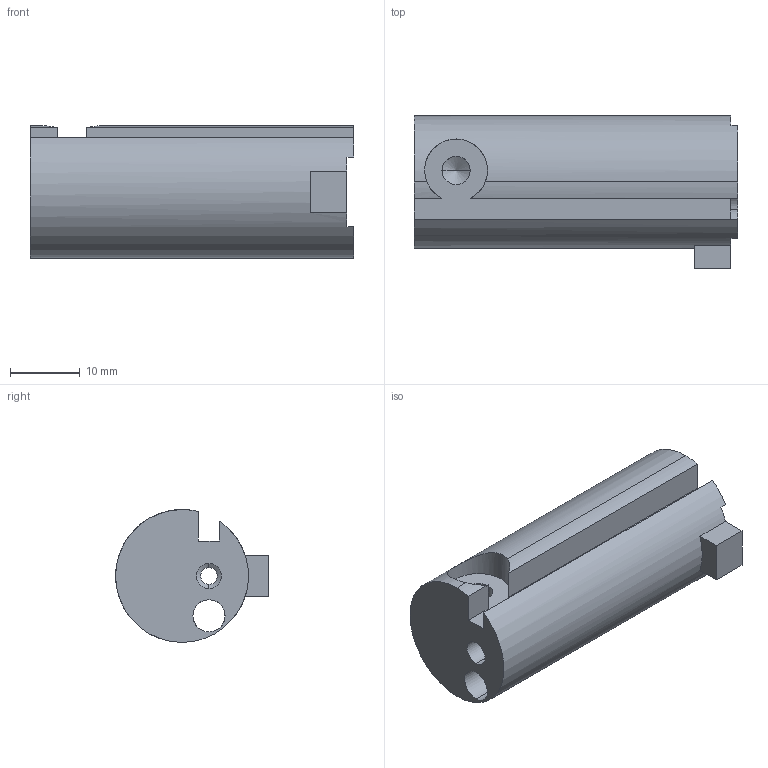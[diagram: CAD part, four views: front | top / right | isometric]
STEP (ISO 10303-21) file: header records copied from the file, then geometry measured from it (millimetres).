
FILE_DESCRIPTION (( 'STEP AP203' ), '1' );
FILE_NAME ('MOD9_V3_Bottom_Bolt.STEP', '2020-12-23T22:01:56', ( '' ), ( '' ), 'SwSTEP 2.0', 'SolidWorks 2019', '' );
FILE_SCHEMA (( 'CONFIG_CONTROL_DESIGN' ));
Length unit declared in the file: millimetre
Products named in the file (1): MOD9_V3_Bottom_Bolt
Bounding box: 46.3 x 21.85 x 19 mm (x, y, z)
Volume: 10922.6 mm3; surface area: 5030.8 mm2
Topology: 1 solids, 1 shells, 34 faces, 91 edges, 57 vertices
Faces by surface type: plane 17, cylinder 13, cone 4
Entity records: 1194 total; most frequent: CARTESIAN_POINT 248, DIRECTION 187, ORIENTED_EDGE 178, EDGE_CURVE 89, AXIS2_PLACEMENT_3D 66, VERTEX_POINT 57, VECTOR 55, LINE 55
